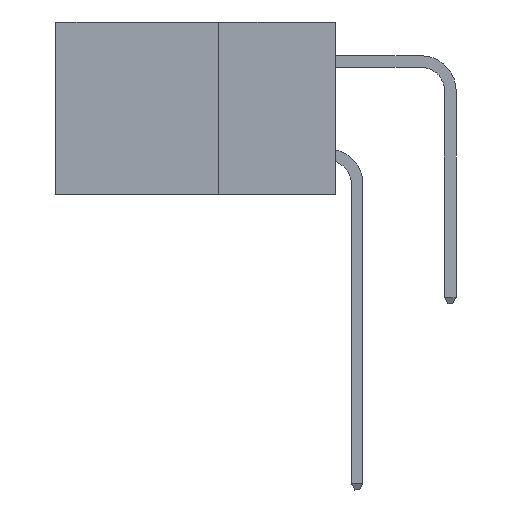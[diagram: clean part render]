
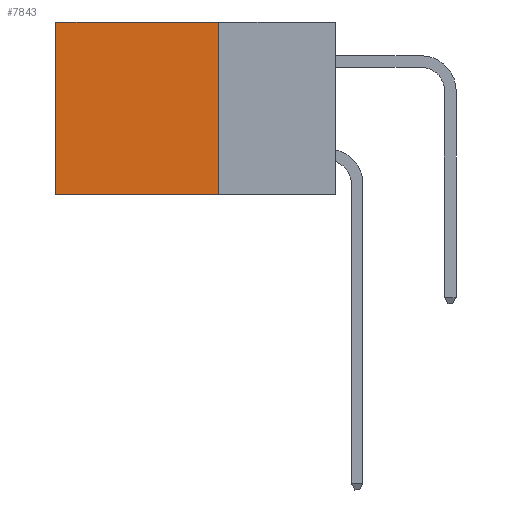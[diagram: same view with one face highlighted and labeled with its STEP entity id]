
A CAD part, left-side view. The second image highlights one B-rep face of the part: STEP entity #7843.
In plain terms, the highlighted planar face has unit normal (-1, 0, 0).
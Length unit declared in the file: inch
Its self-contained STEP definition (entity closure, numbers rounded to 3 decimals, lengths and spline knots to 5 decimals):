
#159 = CARTESIAN_POINT ( 'NONE',  ( 0.2875, 0.25, 0. ) ) ;
#397 = VERTEX_POINT ( 'NONE', #13319 ) ;
#582 = VECTOR ( 'NONE', #2126, 39.37008 ) ;
#1259 = DIRECTION ( 'NONE',  ( 0., 1., 0. ) ) ;
#1395 = CARTESIAN_POINT ( 'NONE',  ( 0.2875, 0.25, 0. ) ) ;
#1959 = EDGE_CURVE ( 'NONE', #7636, #3719, #2899, .T. ) ;
#2108 = CARTESIAN_POINT ( 'NONE',  ( 0.2875, 0.25, 0. ) ) ;
#2126 = DIRECTION ( 'NONE',  ( 0., 0., -1. ) ) ;
#2491 = ORIENTED_EDGE ( 'NONE', *, *, #6123, .T. ) ;
#2899 = LINE ( 'NONE', #10538, #8248 ) ;
#3243 = LINE ( 'NONE', #1395, #8577 ) ;
#3562 = DIRECTION ( 'NONE',  ( 0., 0., -1. ) ) ;
#3607 = CARTESIAN_POINT ( 'NONE',  ( 0.2875, 0.25, -0.37 ) ) ;
#3719 = VERTEX_POINT ( 'NONE', #10107 ) ;
#4841 = LINE ( 'NONE', #159, #13097 ) ;
#6123 = EDGE_CURVE ( 'NONE', #13457, #397, #4841, .T. ) ;
#6678 = EDGE_CURVE ( 'NONE', #397, #3719, #12921, .T. ) ;
#7206 = ORIENTED_EDGE ( 'NONE', *, *, #8176, .F. ) ;
#7435 = DIRECTION ( 'NONE',  ( 0., 0., -1. ) ) ;
#7451 = CARTESIAN_POINT ( 'NONE',  ( 0.2875, 0.6, 0. ) ) ;
#7459 = ORIENTED_EDGE ( 'NONE', *, *, #6678, .T. ) ;
#7636 = VERTEX_POINT ( 'NONE', #3607 ) ;
#7693 = DIRECTION ( 'NONE',  ( 0., 1., 0. ) ) ;
#7843 = ADVANCED_FACE ( 'NONE', ( #8125 ), #10461, .F. ) ;
#8125 = FACE_OUTER_BOUND ( 'NONE', #12209, .T. ) ;
#8170 = ORIENTED_EDGE ( 'NONE', *, *, #1959, .F. ) ;
#8176 = EDGE_CURVE ( 'NONE', #13457, #7636, #3243, .T. ) ;
#8248 = VECTOR ( 'NONE', #7693, 39.37008 ) ;
#8577 = VECTOR ( 'NONE', #3562, 39.37008 ) ;
#8877 = AXIS2_PLACEMENT_3D ( 'NONE', #2108, #10551, #7435 ) ;
#10107 = CARTESIAN_POINT ( 'NONE',  ( 0.2875, 0.6, -0.37 ) ) ;
#10461 = PLANE ( 'NONE',  #8877 ) ;
#10538 = CARTESIAN_POINT ( 'NONE',  ( 0.2875, 0.25, -0.37 ) ) ;
#10551 = DIRECTION ( 'NONE',  ( 1., 0., 0. ) ) ;
#11445 = CARTESIAN_POINT ( 'NONE',  ( 0.2875, 0.25, 0. ) ) ;
#12209 = EDGE_LOOP ( 'NONE', ( #7459, #8170, #7206, #2491 ) ) ;
#12921 = LINE ( 'NONE', #7451, #582 ) ;
#13097 = VECTOR ( 'NONE', #1259, 39.37008 ) ;
#13319 = CARTESIAN_POINT ( 'NONE',  ( 0.2875, 0.6, 0. ) ) ;
#13457 = VERTEX_POINT ( 'NONE', #11445 ) ;
